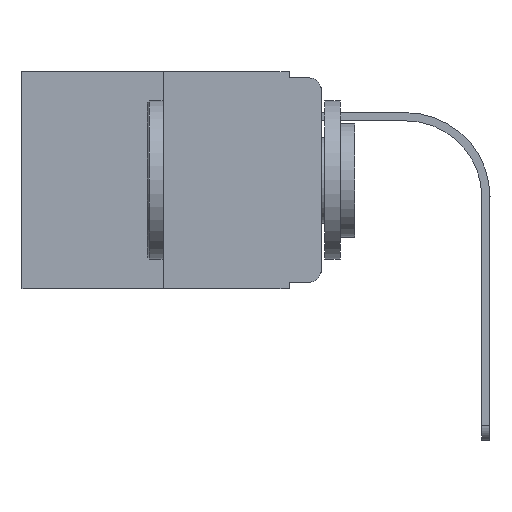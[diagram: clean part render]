
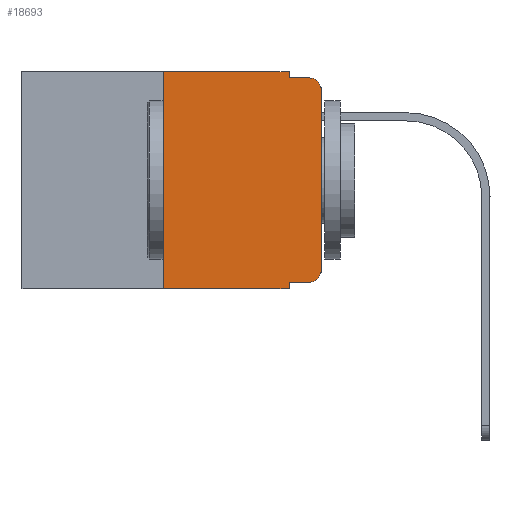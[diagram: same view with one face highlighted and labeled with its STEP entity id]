
A CAD part, left-side view. The second image highlights one B-rep face of the part: STEP entity #18693.
In plain terms, the highlighted planar face has unit normal (-1, 0, 0).
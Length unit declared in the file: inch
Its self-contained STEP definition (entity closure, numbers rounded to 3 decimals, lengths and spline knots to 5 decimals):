
#57 = VERTEX_POINT ( 'NONE', #10062 ) ;
#528 = EDGE_CURVE ( 'NONE', #10285, #57, #9372, .T. ) ;
#588 = EDGE_CURVE ( 'NONE', #12101, #3805, #8058, .T. ) ;
#653 = VECTOR ( 'NONE', #6429, 39.37008 ) ;
#717 = LINE ( 'NONE', #12093, #13861 ) ;
#1313 = VECTOR ( 'NONE', #15706, 39.37008 ) ;
#1444 = CARTESIAN_POINT ( 'NONE',  ( 0., 0., -0.313 ) ) ;
#1450 = VERTEX_POINT ( 'NONE', #3226 ) ;
#1643 = CIRCLE ( 'NONE', #3160, 0.02 ) ;
#2080 = ORIENTED_EDGE ( 'NONE', *, *, #16043, .T. ) ;
#2093 = LINE ( 'NONE', #16359, #5826 ) ;
#2130 = ORIENTED_EDGE ( 'NONE', *, *, #5522, .F. ) ;
#2184 = VERTEX_POINT ( 'NONE', #11350 ) ;
#2434 = CARTESIAN_POINT ( 'NONE',  ( 0., 0.473, 0. ) ) ;
#2712 = VERTEX_POINT ( 'NONE', #1444 ) ;
#3160 = AXIS2_PLACEMENT_3D ( 'NONE', #16896, #12632, #18413 ) ;
#3226 = CARTESIAN_POINT ( 'NONE',  ( 0., 0.02, -0.333 ) ) ;
#3655 = EDGE_LOOP ( 'NONE', ( #2080, #16228, #5728, #12264, #14430, #18335, #14111, #2130, #13313, #3892 ) ) ;
#3719 = LINE ( 'NONE', #11114, #7054 ) ;
#3746 = CARTESIAN_POINT ( 'NONE',  ( 0., 0.25, -0.343 ) ) ;
#3805 = VERTEX_POINT ( 'NONE', #5193 ) ;
#3892 = ORIENTED_EDGE ( 'NONE', *, *, #6685, .T. ) ;
#4762 = VERTEX_POINT ( 'NONE', #11195 ) ;
#5181 = CARTESIAN_POINT ( 'NONE',  ( 0., 0.051, 0. ) ) ;
#5193 = CARTESIAN_POINT ( 'NONE',  ( 0., 0.051, -0.01 ) ) ;
#5325 = CARTESIAN_POINT ( 'NONE',  ( 0., 0.02, -0.01 ) ) ;
#5522 = EDGE_CURVE ( 'NONE', #2184, #57, #5820, .T. ) ;
#5705 = DIRECTION ( 'NONE',  ( 0., -1., 0. ) ) ;
#5728 = ORIENTED_EDGE ( 'NONE', *, *, #12760, .F. ) ;
#5804 = CARTESIAN_POINT ( 'NONE',  ( 0., 0.473, -0.343 ) ) ;
#5820 = LINE ( 'NONE', #10137, #9030 ) ;
#5826 = VECTOR ( 'NONE', #7679, 39.37008 ) ;
#5967 = VERTEX_POINT ( 'NONE', #7301 ) ;
#6429 = DIRECTION ( 'NONE',  ( 0., 0., -1. ) ) ;
#6452 = VECTOR ( 'NONE', #5705, 39.37008 ) ;
#6685 = EDGE_CURVE ( 'NONE', #1450, #2712, #1643, .T. ) ;
#6789 = AXIS2_PLACEMENT_3D ( 'NONE', #8386, #9822, #16862 ) ;
#6862 = PLANE ( 'NONE',  #10873 ) ;
#7054 = VECTOR ( 'NONE', #7844, 39.37008 ) ;
#7301 = CARTESIAN_POINT ( 'NONE',  ( 0., 0., -0.03 ) ) ;
#7679 = DIRECTION ( 'NONE',  ( 0., 0., 1. ) ) ;
#7700 = VECTOR ( 'NONE', #14898, 39.37008 ) ;
#7844 = DIRECTION ( 'NONE',  ( 0., -1., 0. ) ) ;
#8058 = LINE ( 'NONE', #5181, #653 ) ;
#8386 = CARTESIAN_POINT ( 'NONE',  ( 0., 0.02, -0.03 ) ) ;
#9030 = VECTOR ( 'NONE', #18584, 39.37008 ) ;
#9372 = LINE ( 'NONE', #5804, #6452 ) ;
#9822 = DIRECTION ( 'NONE',  ( -1., 0., 0. ) ) ;
#10062 = CARTESIAN_POINT ( 'NONE',  ( 0., 0.051, -0.343 ) ) ;
#10137 = CARTESIAN_POINT ( 'NONE',  ( 0., 0.051, 0. ) ) ;
#10285 = VERTEX_POINT ( 'NONE', #3746 ) ;
#10480 = EDGE_CURVE ( 'NONE', #4762, #12101, #12941, .T. ) ;
#10578 = DIRECTION ( 'NONE',  ( 0., 0., 1. ) ) ;
#10873 = AXIS2_PLACEMENT_3D ( 'NONE', #2434, #12884, #18657 ) ;
#11078 = FACE_OUTER_BOUND ( 'NONE', #3655, .T. ) ;
#11114 = CARTESIAN_POINT ( 'NONE',  ( 0., 0.051, -0.333 ) ) ;
#11195 = CARTESIAN_POINT ( 'NONE',  ( 0., 0.25, 0. ) ) ;
#11350 = CARTESIAN_POINT ( 'NONE',  ( 0., 0.051, -0.333 ) ) ;
#11970 = CIRCLE ( 'NONE', #6789, 0.02 ) ;
#12093 = CARTESIAN_POINT ( 'NONE',  ( 0., 0.25, 0. ) ) ;
#12101 = VERTEX_POINT ( 'NONE', #14462 ) ;
#12264 = ORIENTED_EDGE ( 'NONE', *, *, #588, .F. ) ;
#12632 = DIRECTION ( 'NONE',  ( -1., 0., 0. ) ) ;
#12760 = EDGE_CURVE ( 'NONE', #3805, #13954, #14707, .T. ) ;
#12884 = DIRECTION ( 'NONE',  ( 1., 0., 0. ) ) ;
#12941 = LINE ( 'NONE', #14648, #1313 ) ;
#13313 = ORIENTED_EDGE ( 'NONE', *, *, #13626, .T. ) ;
#13626 = EDGE_CURVE ( 'NONE', #2184, #1450, #3719, .T. ) ;
#13861 = VECTOR ( 'NONE', #10578, 39.37008 ) ;
#13902 = EDGE_CURVE ( 'NONE', #5967, #13954, #11970, .T. ) ;
#13954 = VERTEX_POINT ( 'NONE', #5325 ) ;
#14111 = ORIENTED_EDGE ( 'NONE', *, *, #528, .T. ) ;
#14190 = EDGE_CURVE ( 'NONE', #10285, #4762, #717, .T. ) ;
#14430 = ORIENTED_EDGE ( 'NONE', *, *, #10480, .F. ) ;
#14462 = CARTESIAN_POINT ( 'NONE',  ( 0., 0.051, 0. ) ) ;
#14648 = CARTESIAN_POINT ( 'NONE',  ( 0., 0.473, 0. ) ) ;
#14707 = LINE ( 'NONE', #16214, #7700 ) ;
#14898 = DIRECTION ( 'NONE',  ( 0., -1., 0. ) ) ;
#15706 = DIRECTION ( 'NONE',  ( 0., -1., 0. ) ) ;
#16043 = EDGE_CURVE ( 'NONE', #2712, #5967, #2093, .T. ) ;
#16214 = CARTESIAN_POINT ( 'NONE',  ( 0., 0.051, -0.01 ) ) ;
#16228 = ORIENTED_EDGE ( 'NONE', *, *, #13902, .T. ) ;
#16359 = CARTESIAN_POINT ( 'NONE',  ( 0., 0., 0. ) ) ;
#16862 = DIRECTION ( 'NONE',  ( 0., 0., -1. ) ) ;
#16896 = CARTESIAN_POINT ( 'NONE',  ( 0., 0.02, -0.313 ) ) ;
#18335 = ORIENTED_EDGE ( 'NONE', *, *, #14190, .F. ) ;
#18413 = DIRECTION ( 'NONE',  ( 0., 0., -1. ) ) ;
#18584 = DIRECTION ( 'NONE',  ( 0., 0., -1. ) ) ;
#18657 = DIRECTION ( 'NONE',  ( 0., 0., -1. ) ) ;
#18693 = ADVANCED_FACE ( 'NONE', ( #11078 ), #6862, .F. ) ;
